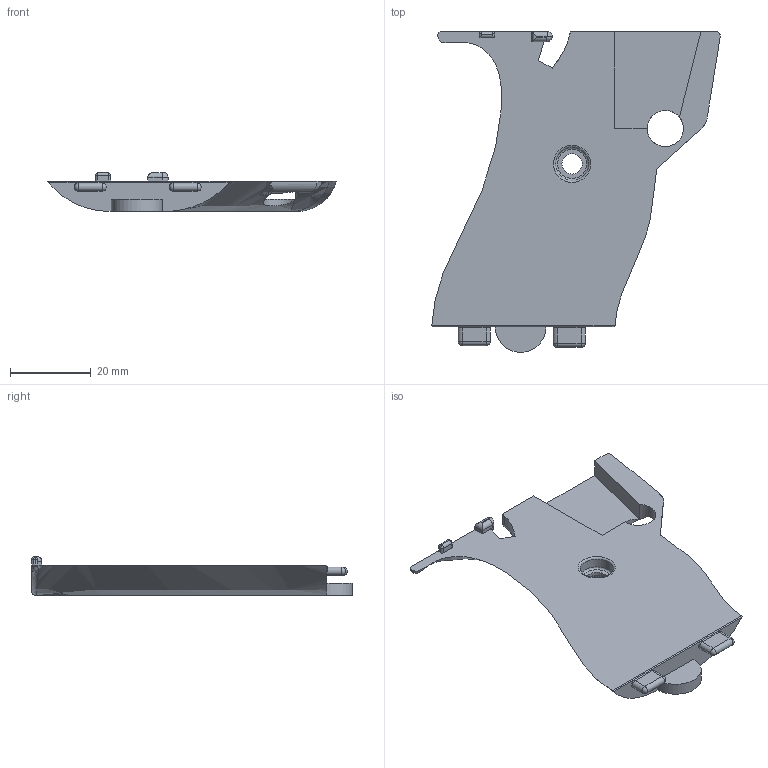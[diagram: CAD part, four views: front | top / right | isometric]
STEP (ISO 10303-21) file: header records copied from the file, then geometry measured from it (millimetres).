
FILE_DESCRIPTION(/* description */ (''),/* implementation_level */ '2;1');
FILE_NAME(/* name */ 'Freeman1337-lopoint-grip-L.step',/* time_stamp */ '2021-05-10T14:43:48-07:00',/* author */ (''),/* organization */ (''),/* preprocessor_version */ 'ST-DEVELOPER v18.1',/* originating_system */ 'Autodesk Translation Framework v10.6.0.1341',/* authorisation */ '');
FILE_SCHEMA (('AUTOMOTIVE_DESIGN { 1 0 10303 214 3 1 1 }'));
Products named in the file (1): Freeman1337-lopoint-grip-L
Bounding box: 71.37 x 79.3 x 9.6 mm (x, y, z)
Volume: 18150.8 mm3; surface area: 8813.8 mm2
Topology: 3 solids, 3 shells, 1698 faces, 4774 edges, 3156 vertices
Faces by surface type: bspline 1398, plane 239, cylinder 45, torus 11, sphere 5
Full cylindrical faces by diameter (mm): 4.472 x1, 5 x1, 8.2 x2, 8.985 x1
Entity records: 60300 total; most frequent: CARTESIAN_POINT 30141, ORIENTED_EDGE 9532, EDGE_CURVE 4766, VERTEX_POINT 3156, DIRECTION 2665, LINE 1817, VECTOR 1817, EDGE_LOOP 1785
